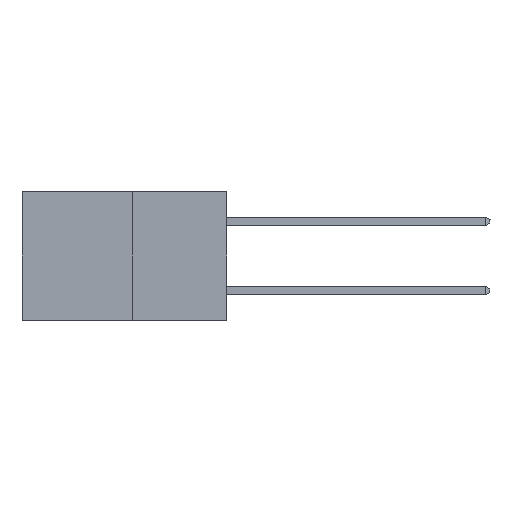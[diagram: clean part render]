
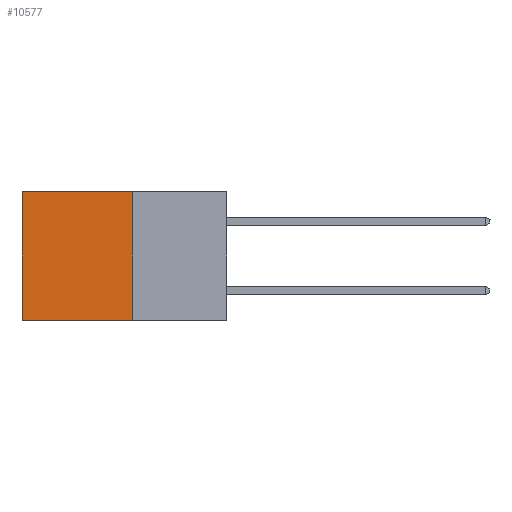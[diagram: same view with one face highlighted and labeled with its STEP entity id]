
A CAD part, left-side view. The second image highlights one B-rep face of the part: STEP entity #10577.
In plain terms, the highlighted planar face has unit normal (-1, 0, 0).
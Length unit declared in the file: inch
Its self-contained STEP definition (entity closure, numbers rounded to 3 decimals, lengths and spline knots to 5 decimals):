
#6 = LINE ( 'NONE', #6471, #8120 ) ;
#232 = VERTEX_POINT ( 'NONE', #6323 ) ;
#1627 = VECTOR ( 'NONE', #2156, 39.37008 ) ;
#1761 = DIRECTION ( 'NONE',  ( 0., 1., 0. ) ) ;
#2156 = DIRECTION ( 'NONE',  ( 0., 0., -1. ) ) ;
#3094 = AXIS2_PLACEMENT_3D ( 'NONE', #9846, #4549, #11936 ) ;
#3474 = PLANE ( 'NONE',  #3094 ) ;
#4438 = EDGE_CURVE ( 'NONE', #5987, #232, #10165, .T. ) ;
#4549 = DIRECTION ( 'NONE',  ( 1., 0., 0. ) ) ;
#4922 = LINE ( 'NONE', #5781, #11192 ) ;
#4985 = CARTESIAN_POINT ( 'NONE',  ( 0.277, 0.27, -0.37 ) ) ;
#5540 = VERTEX_POINT ( 'NONE', #9899 ) ;
#5781 = CARTESIAN_POINT ( 'NONE',  ( 0.277, 0.27, 0. ) ) ;
#5987 = VERTEX_POINT ( 'NONE', #9104 ) ;
#6323 = CARTESIAN_POINT ( 'NONE',  ( 0.277, 0.59, -0.37 ) ) ;
#6471 = CARTESIAN_POINT ( 'NONE',  ( 0.277, 0.59, -0.37 ) ) ;
#7244 = ORIENTED_EDGE ( 'NONE', *, *, #4438, .F. ) ;
#7414 = VECTOR ( 'NONE', #1761, 39.37008 ) ;
#7606 = LINE ( 'NONE', #11612, #1627 ) ;
#8120 = VECTOR ( 'NONE', #8568, 39.37008 ) ;
#8156 = ORIENTED_EDGE ( 'NONE', *, *, #12896, .T. ) ;
#8568 = DIRECTION ( 'NONE',  ( 0., 0., -1. ) ) ;
#8965 = EDGE_CURVE ( 'NONE', #13385, #232, #6, .T. ) ;
#9104 = CARTESIAN_POINT ( 'NONE',  ( 0.277, 0.27, -0.37 ) ) ;
#9668 = EDGE_CURVE ( 'NONE', #5540, #5987, #7606, .T. ) ;
#9740 = ORIENTED_EDGE ( 'NONE', *, *, #8965, .T. ) ;
#9822 = ORIENTED_EDGE ( 'NONE', *, *, #9668, .F. ) ;
#9846 = CARTESIAN_POINT ( 'NONE',  ( 0.277, 0.27, -0.37 ) ) ;
#9899 = CARTESIAN_POINT ( 'NONE',  ( 0.277, 0.27, 0. ) ) ;
#10165 = LINE ( 'NONE', #4985, #7414 ) ;
#10577 = ADVANCED_FACE ( 'NONE', ( #13518 ), #3474, .F. ) ;
#11121 = EDGE_LOOP ( 'NONE', ( #9740, #7244, #9822, #8156 ) ) ;
#11192 = VECTOR ( 'NONE', #13100, 39.37008 ) ;
#11612 = CARTESIAN_POINT ( 'NONE',  ( 0.277, 0.27, -0.37 ) ) ;
#11936 = DIRECTION ( 'NONE',  ( 0., 0., -1. ) ) ;
#12763 = CARTESIAN_POINT ( 'NONE',  ( 0.277, 0.59, 0. ) ) ;
#12896 = EDGE_CURVE ( 'NONE', #5540, #13385, #4922, .T. ) ;
#13100 = DIRECTION ( 'NONE',  ( 0., 1., 0. ) ) ;
#13385 = VERTEX_POINT ( 'NONE', #12763 ) ;
#13518 = FACE_OUTER_BOUND ( 'NONE', #11121, .T. ) ;
